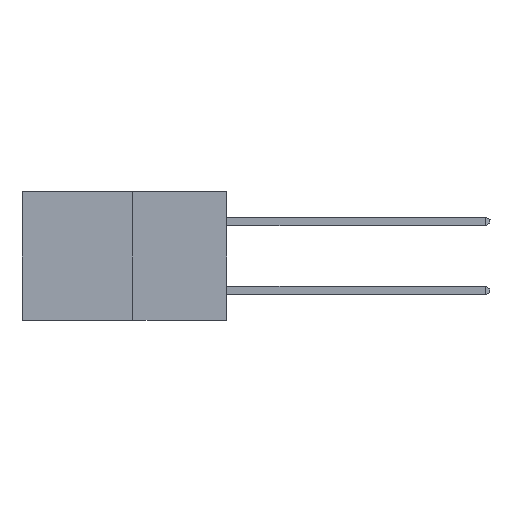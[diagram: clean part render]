
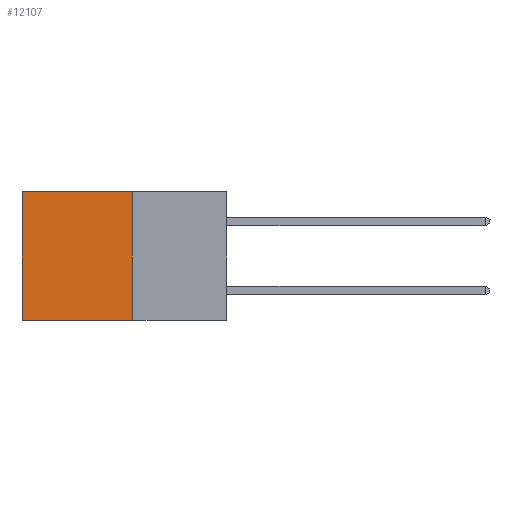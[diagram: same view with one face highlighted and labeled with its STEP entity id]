
A CAD part, left-side view. The second image highlights one B-rep face of the part: STEP entity #12107.
In plain terms, the highlighted planar face has unit normal (-1, 0, 0).
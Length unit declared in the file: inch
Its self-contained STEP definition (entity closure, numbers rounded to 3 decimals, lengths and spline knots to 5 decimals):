
#128 = CARTESIAN_POINT ( 'NONE',  ( 0.277, 0.27, -0.37 ) ) ;
#497 = EDGE_CURVE ( 'NONE', #23250, #13515, #11195, .T. ) ;
#1100 = ORIENTED_EDGE ( 'NONE', *, *, #497, .T. ) ;
#1908 = EDGE_CURVE ( 'NONE', #12025, #13515, #10186, .T. ) ;
#2466 = PLANE ( 'NONE',  #5043 ) ;
#2661 = VECTOR ( 'NONE', #21662, 39.37008 ) ;
#4555 = DIRECTION ( 'NONE',  ( 0., 0., -1. ) ) ;
#5043 = AXIS2_PLACEMENT_3D ( 'NONE', #18576, #16729, #4555 ) ;
#5468 = VECTOR ( 'NONE', #10148, 39.37008 ) ;
#7260 = ORIENTED_EDGE ( 'NONE', *, *, #19053, .F. ) ;
#8141 = LINE ( 'NONE', #13889, #2661 ) ;
#8659 = EDGE_LOOP ( 'NONE', ( #1100, #17363, #7260, #23082 ) ) ;
#9567 = CARTESIAN_POINT ( 'NONE',  ( 0.277, 0.27, 0. ) ) ;
#10148 = DIRECTION ( 'NONE',  ( 0., 1., 0. ) ) ;
#10186 = LINE ( 'NONE', #16539, #15562 ) ;
#11195 = LINE ( 'NONE', #22944, #21061 ) ;
#12025 = VERTEX_POINT ( 'NONE', #128 ) ;
#12107 = ADVANCED_FACE ( 'NONE', ( #14962 ), #2466, .F. ) ;
#13515 = VERTEX_POINT ( 'NONE', #23135 ) ;
#13889 = CARTESIAN_POINT ( 'NONE',  ( 0.277, 0.27, -0.37 ) ) ;
#14962 = FACE_OUTER_BOUND ( 'NONE', #8659, .T. ) ;
#15562 = VECTOR ( 'NONE', #19383, 39.37008 ) ;
#16539 = CARTESIAN_POINT ( 'NONE',  ( 0.277, 0.27, -0.37 ) ) ;
#16729 = DIRECTION ( 'NONE',  ( 1., 0., 0. ) ) ;
#17363 = ORIENTED_EDGE ( 'NONE', *, *, #1908, .F. ) ;
#18083 = CARTESIAN_POINT ( 'NONE',  ( 0.277, 0.27, 0. ) ) ;
#18398 = DIRECTION ( 'NONE',  ( 0., 0., -1. ) ) ;
#18576 = CARTESIAN_POINT ( 'NONE',  ( 0.277, 0.27, -0.37 ) ) ;
#19053 = EDGE_CURVE ( 'NONE', #24283, #12025, #8141, .T. ) ;
#19383 = DIRECTION ( 'NONE',  ( 0., 1., 0. ) ) ;
#21061 = VECTOR ( 'NONE', #18398, 39.37008 ) ;
#21405 = LINE ( 'NONE', #18083, #5468 ) ;
#21662 = DIRECTION ( 'NONE',  ( 0., 0., -1. ) ) ;
#22047 = CARTESIAN_POINT ( 'NONE',  ( 0.277, 0.59, 0. ) ) ;
#22944 = CARTESIAN_POINT ( 'NONE',  ( 0.277, 0.59, -0.37 ) ) ;
#23082 = ORIENTED_EDGE ( 'NONE', *, *, #25156, .T. ) ;
#23135 = CARTESIAN_POINT ( 'NONE',  ( 0.277, 0.59, -0.37 ) ) ;
#23250 = VERTEX_POINT ( 'NONE', #22047 ) ;
#24283 = VERTEX_POINT ( 'NONE', #9567 ) ;
#25156 = EDGE_CURVE ( 'NONE', #24283, #23250, #21405, .T. ) ;
